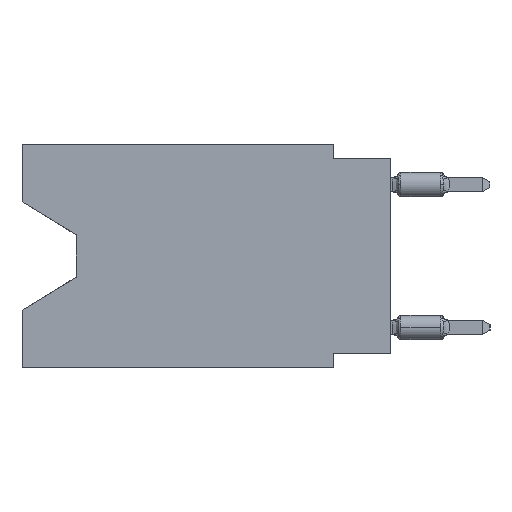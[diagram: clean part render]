
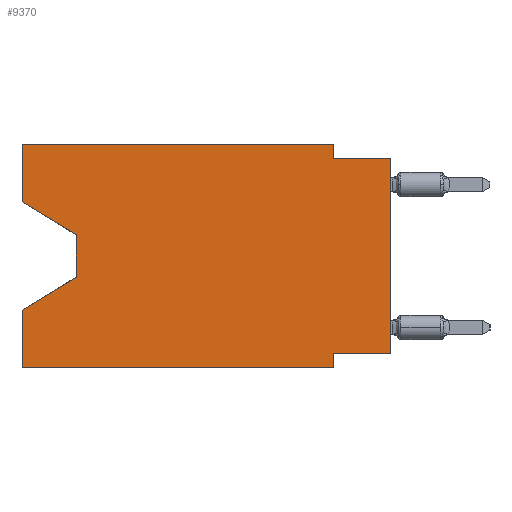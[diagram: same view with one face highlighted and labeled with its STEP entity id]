
A CAD part, left-side view. The second image highlights one B-rep face of the part: STEP entity #9370.
In plain terms, the highlighted planar face has unit normal (-1, 0, 0).
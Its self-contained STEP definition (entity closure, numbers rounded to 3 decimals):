
#489 = CARTESIAN_POINT ( 'NONE',  ( 0., 2.54, 0. ) ) ;
#708 = CARTESIAN_POINT ( 'NONE',  ( 0., 16.383, 0. ) ) ;
#2074 = CARTESIAN_POINT ( 'NONE',  ( 0., 13.97, -5.893 ) ) ;
#3573 = EDGE_CURVE ( 'NONE', #23919, #22327, #6181, .T. ) ;
#4347 = DIRECTION ( 'NONE',  ( 0., -1., 0. ) ) ;
#4552 = DIRECTION ( 'NONE',  ( 0., 0.855, -0.519 ) ) ;
#4696 = VERTEX_POINT ( 'NONE', #30672 ) ;
#4898 = VECTOR ( 'NONE', #4347, 1000. ) ;
#5551 = DIRECTION ( 'NONE',  ( 0., 0., 1. ) ) ;
#5787 = VECTOR ( 'NONE', #26365, 1000. ) ;
#6009 = EDGE_CURVE ( 'NONE', #4696, #12941, #31948, .T. ) ;
#6181 = LINE ( 'NONE', #25775, #34114 ) ;
#6216 = VERTEX_POINT ( 'NONE', #33975 ) ;
#6455 = EDGE_CURVE ( 'NONE', #31457, #7803, #27511, .T. ) ;
#7803 = VERTEX_POINT ( 'NONE', #45758 ) ;
#8263 = VERTEX_POINT ( 'NONE', #25069 ) ;
#9370 = ADVANCED_FACE ( 'NONE', ( #31092 ), #24628, .F. ) ;
#10140 = EDGE_CURVE ( 'NONE', #12583, #47204, #23946, .T. ) ;
#11523 = CARTESIAN_POINT ( 'NONE',  ( 0., 2.54, -9.906 ) ) ;
#12406 = ORIENTED_EDGE ( 'NONE', *, *, #6009, .T. ) ;
#12537 = LINE ( 'NONE', #40645, #32530 ) ;
#12583 = VERTEX_POINT ( 'NONE', #27793 ) ;
#12941 = VERTEX_POINT ( 'NONE', #32806 ) ;
#14451 = ORIENTED_EDGE ( 'NONE', *, *, #26379, .T. ) ;
#15117 = VECTOR ( 'NONE', #5551, 1000. ) ;
#15652 = DIRECTION ( 'NONE',  ( 0., 0., -1. ) ) ;
#16619 = EDGE_LOOP ( 'NONE', ( #14451, #37160, #45221, #42393, #45094, #40854, #23738, #12406, #30684, #30205, #34684, #48416 ) ) ;
#17408 = DIRECTION ( 'NONE',  ( 1., 0., 0. ) ) ;
#17735 = CARTESIAN_POINT ( 'NONE',  ( 0., 13.97, -4.013 ) ) ;
#18121 = LINE ( 'NONE', #26617, #5787 ) ;
#20036 = DIRECTION ( 'NONE',  ( 0., 0., 1. ) ) ;
#20514 = DIRECTION ( 'NONE',  ( 0., 0., -1. ) ) ;
#21162 = CARTESIAN_POINT ( 'NONE',  ( 0., 2.54, -9.271 ) ) ;
#21506 = VECTOR ( 'NONE', #34060, 1000. ) ;
#21527 = LINE ( 'NONE', #26427, #15117 ) ;
#22327 = VERTEX_POINT ( 'NONE', #2074 ) ;
#22535 = CARTESIAN_POINT ( 'NONE',  ( 0., 2.54, -0.635 ) ) ;
#23170 = CARTESIAN_POINT ( 'NONE',  ( 0., 16.383, -9.906 ) ) ;
#23643 = CARTESIAN_POINT ( 'NONE',  ( 0., 16.383, 0. ) ) ;
#23738 = ORIENTED_EDGE ( 'NONE', *, *, #49358, .F. ) ;
#23919 = VERTEX_POINT ( 'NONE', #17735 ) ;
#23946 = LINE ( 'NONE', #708, #4898 ) ;
#24627 = AXIS2_PLACEMENT_3D ( 'NONE', #28752, #17408, #20514 ) ;
#24628 = PLANE ( 'NONE',  #24627 ) ;
#24829 = CARTESIAN_POINT ( 'NONE',  ( 0., 2.54, 0. ) ) ;
#25069 = CARTESIAN_POINT ( 'NONE',  ( 0., 16.383, -9.906 ) ) ;
#25775 = CARTESIAN_POINT ( 'NONE',  ( 0., 13.97, -4.013 ) ) ;
#25809 = CARTESIAN_POINT ( 'NONE',  ( 0., 0., -9.271 ) ) ;
#26322 = LINE ( 'NONE', #25809, #21506 ) ;
#26365 = DIRECTION ( 'NONE',  ( 0., -1., 0. ) ) ;
#26379 = EDGE_CURVE ( 'NONE', #6216, #23919, #38854, .T. ) ;
#26427 = CARTESIAN_POINT ( 'NONE',  ( 0., 16.383, 0. ) ) ;
#26617 = CARTESIAN_POINT ( 'NONE',  ( 0., 0., -0.635 ) ) ;
#27511 = LINE ( 'NONE', #11523, #46846 ) ;
#27793 = CARTESIAN_POINT ( 'NONE',  ( 0., 16.383, 0. ) ) ;
#28752 = CARTESIAN_POINT ( 'NONE',  ( 0., 16.383, 0. ) ) ;
#29096 = VECTOR ( 'NONE', #20036, 1000. ) ;
#29440 = EDGE_CURVE ( 'NONE', #6216, #12583, #21527, .T. ) ;
#30205 = ORIENTED_EDGE ( 'NONE', *, *, #42153, .F. ) ;
#30380 = VERTEX_POINT ( 'NONE', #42306 ) ;
#30672 = CARTESIAN_POINT ( 'NONE',  ( 0., 0., -9.271 ) ) ;
#30684 = ORIENTED_EDGE ( 'NONE', *, *, #46936, .F. ) ;
#30916 = DIRECTION ( 'NONE',  ( 0., -1., 0. ) ) ;
#30961 = EDGE_CURVE ( 'NONE', #8263, #30380, #39624, .T. ) ;
#31092 = FACE_OUTER_BOUND ( 'NONE', #16619, .T. ) ;
#31457 = VERTEX_POINT ( 'NONE', #21162 ) ;
#31948 = LINE ( 'NONE', #35829, #36896 ) ;
#32317 = LINE ( 'NONE', #24829, #50777 ) ;
#32365 = EDGE_CURVE ( 'NONE', #22327, #30380, #12537, .T. ) ;
#32530 = VECTOR ( 'NONE', #4552, 1000. ) ;
#32806 = CARTESIAN_POINT ( 'NONE',  ( 0., 0., -0.635 ) ) ;
#33975 = CARTESIAN_POINT ( 'NONE',  ( 0., 16.383, -2.546 ) ) ;
#34060 = DIRECTION ( 'NONE',  ( 0., 1., 0. ) ) ;
#34114 = VECTOR ( 'NONE', #49530, 1000. ) ;
#34684 = ORIENTED_EDGE ( 'NONE', *, *, #10140, .F. ) ;
#35829 = CARTESIAN_POINT ( 'NONE',  ( 0., 0., 0. ) ) ;
#36071 = DIRECTION ( 'NONE',  ( 0., 0., 1. ) ) ;
#36191 = EDGE_CURVE ( 'NONE', #8263, #7803, #50532, .T. ) ;
#36896 = VECTOR ( 'NONE', #36071, 1000. ) ;
#37160 = ORIENTED_EDGE ( 'NONE', *, *, #3573, .T. ) ;
#38854 = LINE ( 'NONE', #43261, #44335 ) ;
#39624 = LINE ( 'NONE', #23643, #29096 ) ;
#40615 = VERTEX_POINT ( 'NONE', #22535 ) ;
#40645 = CARTESIAN_POINT ( 'NONE',  ( 0., 13.97, -5.893 ) ) ;
#40854 = ORIENTED_EDGE ( 'NONE', *, *, #6455, .F. ) ;
#41104 = VECTOR ( 'NONE', #30916, 1000. ) ;
#42153 = EDGE_CURVE ( 'NONE', #47204, #40615, #32317, .T. ) ;
#42306 = CARTESIAN_POINT ( 'NONE',  ( 0., 16.383, -7.36 ) ) ;
#42393 = ORIENTED_EDGE ( 'NONE', *, *, #30961, .F. ) ;
#42998 = DIRECTION ( 'NONE',  ( 0., -0.855, -0.519 ) ) ;
#43261 = CARTESIAN_POINT ( 'NONE',  ( 0., 16.383, -2.546 ) ) ;
#44335 = VECTOR ( 'NONE', #42998, 1000. ) ;
#45094 = ORIENTED_EDGE ( 'NONE', *, *, #36191, .T. ) ;
#45221 = ORIENTED_EDGE ( 'NONE', *, *, #32365, .T. ) ;
#45758 = CARTESIAN_POINT ( 'NONE',  ( 0., 2.54, -9.906 ) ) ;
#46846 = VECTOR ( 'NONE', #15652, 1000. ) ;
#46936 = EDGE_CURVE ( 'NONE', #40615, #12941, #18121, .T. ) ;
#47204 = VERTEX_POINT ( 'NONE', #489 ) ;
#48416 = ORIENTED_EDGE ( 'NONE', *, *, #29440, .F. ) ;
#48825 = DIRECTION ( 'NONE',  ( 0., 0., -1. ) ) ;
#49358 = EDGE_CURVE ( 'NONE', #4696, #31457, #26322, .T. ) ;
#49530 = DIRECTION ( 'NONE',  ( 0., 0., -1. ) ) ;
#50532 = LINE ( 'NONE', #23170, #41104 ) ;
#50777 = VECTOR ( 'NONE', #48825, 1000. ) ;
